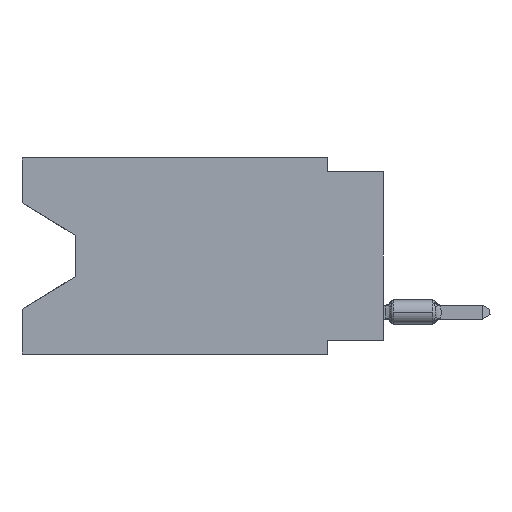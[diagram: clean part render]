
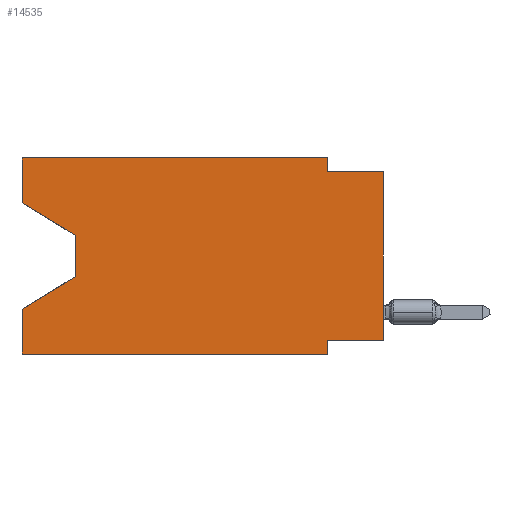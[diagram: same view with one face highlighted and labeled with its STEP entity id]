
A CAD part, left-side view. The second image highlights one B-rep face of the part: STEP entity #14535.
In plain terms, the highlighted planar face has unit normal (-1, 0, 0).
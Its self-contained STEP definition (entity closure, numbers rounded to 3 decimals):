
#189 = CARTESIAN_POINT ( 'NONE',  ( 0., 2.54, -8.89 ) ) ;
#1152 = DIRECTION ( 'NONE',  ( 0., -1., 0. ) ) ;
#1521 = VECTOR ( 'NONE', #8471, 1000. ) ;
#1672 = LINE ( 'NONE', #10391, #28402 ) ;
#2372 = PLANE ( 'NONE',  #4745 ) ;
#2667 = EDGE_CURVE ( 'NONE', #40675, #30072, #1672, .T. ) ;
#2773 = CARTESIAN_POINT ( 'NONE',  ( 0., 2.54, -8.255 ) ) ;
#2877 = DIRECTION ( 'NONE',  ( 0., 0., 1. ) ) ;
#3129 = ORIENTED_EDGE ( 'NONE', *, *, #21490, .F. ) ;
#3187 = VECTOR ( 'NONE', #12646, 1000. ) ;
#3313 = EDGE_LOOP ( 'NONE', ( #17194, #50690, #22712, #18168, #48537, #9371, #3129, #34352, #26131, #28840, #4667, #29507 ) ) ;
#4667 = ORIENTED_EDGE ( 'NONE', *, *, #45572, .F. ) ;
#4745 = AXIS2_PLACEMENT_3D ( 'NONE', #51872, #55062, #33924 ) ;
#5497 = CARTESIAN_POINT ( 'NONE',  ( 0., 16.383, 0. ) ) ;
#5657 = VERTEX_POINT ( 'NONE', #47585 ) ;
#6975 = CARTESIAN_POINT ( 'NONE',  ( 0., 16.383, -8.89 ) ) ;
#8471 = DIRECTION ( 'NONE',  ( 0., 0., -1. ) ) ;
#9371 = ORIENTED_EDGE ( 'NONE', *, *, #18249, .F. ) ;
#10048 = CARTESIAN_POINT ( 'NONE',  ( 0., 2.54, -0.635 ) ) ;
#10391 = CARTESIAN_POINT ( 'NONE',  ( 0., 16.383, -8.89 ) ) ;
#10810 = VERTEX_POINT ( 'NONE', #30457 ) ;
#11039 = VERTEX_POINT ( 'NONE', #33581 ) ;
#11917 = VECTOR ( 'NONE', #31040, 1000. ) ;
#12646 = DIRECTION ( 'NONE',  ( 0., 0., -1. ) ) ;
#13385 = CARTESIAN_POINT ( 'NONE',  ( 0., 0., 0. ) ) ;
#14535 = ADVANCED_FACE ( 'NONE', ( #37704 ), #2372, .F. ) ;
#15338 = DIRECTION ( 'NONE',  ( 0., 1., 0. ) ) ;
#15659 = DIRECTION ( 'NONE',  ( 0., 0.855, -0.519 ) ) ;
#16528 = CARTESIAN_POINT ( 'NONE',  ( 0., 16.383, 0. ) ) ;
#17123 = VECTOR ( 'NONE', #44766, 1000. ) ;
#17194 = ORIENTED_EDGE ( 'NONE', *, *, #47221, .T. ) ;
#17737 = CARTESIAN_POINT ( 'NONE',  ( 0., 13.97, -3.505 ) ) ;
#18168 = ORIENTED_EDGE ( 'NONE', *, *, #37166, .F. ) ;
#18249 = EDGE_CURVE ( 'NONE', #38470, #30072, #25974, .T. ) ;
#18782 = VECTOR ( 'NONE', #15338, 1000. ) ;
#19729 = VECTOR ( 'NONE', #2877, 1000. ) ;
#20271 = CARTESIAN_POINT ( 'NONE',  ( 0., 0., -8.255 ) ) ;
#20915 = VECTOR ( 'NONE', #29860, 1000. ) ;
#21427 = EDGE_CURVE ( 'NONE', #11039, #5657, #24601, .T. ) ;
#21490 = EDGE_CURVE ( 'NONE', #45180, #38470, #50933, .T. ) ;
#21503 = LINE ( 'NONE', #17737, #1521 ) ;
#22232 = VECTOR ( 'NONE', #1152, 1000. ) ;
#22712 = ORIENTED_EDGE ( 'NONE', *, *, #53117, .T. ) ;
#23623 = VECTOR ( 'NONE', #15659, 1000. ) ;
#24099 = LINE ( 'NONE', #41746, #36102 ) ;
#24326 = CARTESIAN_POINT ( 'NONE',  ( 0., 0., -8.255 ) ) ;
#24601 = LINE ( 'NONE', #41392, #19729 ) ;
#25974 = LINE ( 'NONE', #189, #3187 ) ;
#26131 = ORIENTED_EDGE ( 'NONE', *, *, #54089, .F. ) ;
#26670 = VECTOR ( 'NONE', #49909, 1000. ) ;
#27122 = CARTESIAN_POINT ( 'NONE',  ( 0., 0., -0.635 ) ) ;
#27637 = CARTESIAN_POINT ( 'NONE',  ( 0., 2.54, 0. ) ) ;
#28098 = VERTEX_POINT ( 'NONE', #29955 ) ;
#28402 = VECTOR ( 'NONE', #55216, 1000. ) ;
#28840 = ORIENTED_EDGE ( 'NONE', *, *, #39466, .F. ) ;
#29507 = ORIENTED_EDGE ( 'NONE', *, *, #21427, .F. ) ;
#29860 = DIRECTION ( 'NONE',  ( 0., 0., 1. ) ) ;
#29955 = CARTESIAN_POINT ( 'NONE',  ( 0., 13.97, -3.505 ) ) ;
#30072 = VERTEX_POINT ( 'NONE', #54925 ) ;
#30457 = CARTESIAN_POINT ( 'NONE',  ( 0., 13.97, -5.385 ) ) ;
#31040 = DIRECTION ( 'NONE',  ( 0., 0., 1. ) ) ;
#32269 = CARTESIAN_POINT ( 'NONE',  ( 0., 0., -0.635 ) ) ;
#32496 = CARTESIAN_POINT ( 'NONE',  ( 0., 2.54, 0. ) ) ;
#33088 = VERTEX_POINT ( 'NONE', #32496 ) ;
#33581 = CARTESIAN_POINT ( 'NONE',  ( 0., 16.383, -2.038 ) ) ;
#33924 = DIRECTION ( 'NONE',  ( 0., 0., -1. ) ) ;
#34352 = ORIENTED_EDGE ( 'NONE', *, *, #43828, .T. ) ;
#35916 = LINE ( 'NONE', #5497, #22232 ) ;
#36102 = VECTOR ( 'NONE', #37409, 1000. ) ;
#36480 = VERTEX_POINT ( 'NONE', #32269 ) ;
#37166 = EDGE_CURVE ( 'NONE', #40675, #47612, #38545, .T. ) ;
#37409 = DIRECTION ( 'NONE',  ( 0., -0.855, -0.519 ) ) ;
#37704 = FACE_OUTER_BOUND ( 'NONE', #3313, .T. ) ;
#38470 = VERTEX_POINT ( 'NONE', #2773 ) ;
#38536 = LINE ( 'NONE', #55303, #23623 ) ;
#38545 = LINE ( 'NONE', #16528, #20915 ) ;
#39466 = EDGE_CURVE ( 'NONE', #33088, #49817, #45577, .T. ) ;
#40675 = VERTEX_POINT ( 'NONE', #6975 ) ;
#41392 = CARTESIAN_POINT ( 'NONE',  ( 0., 16.383, 0. ) ) ;
#41746 = CARTESIAN_POINT ( 'NONE',  ( 0., 16.383, -2.038 ) ) ;
#43828 = EDGE_CURVE ( 'NONE', #45180, #36480, #53873, .T. ) ;
#44151 = CARTESIAN_POINT ( 'NONE',  ( 0., 16.383, -6.852 ) ) ;
#44766 = DIRECTION ( 'NONE',  ( 0., -1., 0. ) ) ;
#45180 = VERTEX_POINT ( 'NONE', #20271 ) ;
#45572 = EDGE_CURVE ( 'NONE', #5657, #33088, #35916, .T. ) ;
#45577 = LINE ( 'NONE', #27637, #26670 ) ;
#47221 = EDGE_CURVE ( 'NONE', #11039, #28098, #24099, .T. ) ;
#47585 = CARTESIAN_POINT ( 'NONE',  ( 0., 16.383, 0. ) ) ;
#47612 = VERTEX_POINT ( 'NONE', #44151 ) ;
#48537 = ORIENTED_EDGE ( 'NONE', *, *, #2667, .T. ) ;
#49817 = VERTEX_POINT ( 'NONE', #10048 ) ;
#49909 = DIRECTION ( 'NONE',  ( 0., 0., -1. ) ) ;
#50690 = ORIENTED_EDGE ( 'NONE', *, *, #56024, .T. ) ;
#50933 = LINE ( 'NONE', #24326, #18782 ) ;
#51872 = CARTESIAN_POINT ( 'NONE',  ( 0., 16.383, 0. ) ) ;
#53117 = EDGE_CURVE ( 'NONE', #10810, #47612, #38536, .T. ) ;
#53873 = LINE ( 'NONE', #13385, #11917 ) ;
#54089 = EDGE_CURVE ( 'NONE', #49817, #36480, #54851, .T. ) ;
#54851 = LINE ( 'NONE', #27122, #17123 ) ;
#54925 = CARTESIAN_POINT ( 'NONE',  ( 0., 2.54, -8.89 ) ) ;
#55062 = DIRECTION ( 'NONE',  ( 1., 0., 0. ) ) ;
#55216 = DIRECTION ( 'NONE',  ( 0., -1., 0. ) ) ;
#55303 = CARTESIAN_POINT ( 'NONE',  ( 0., 13.97, -5.385 ) ) ;
#56024 = EDGE_CURVE ( 'NONE', #28098, #10810, #21503, .T. ) ;
